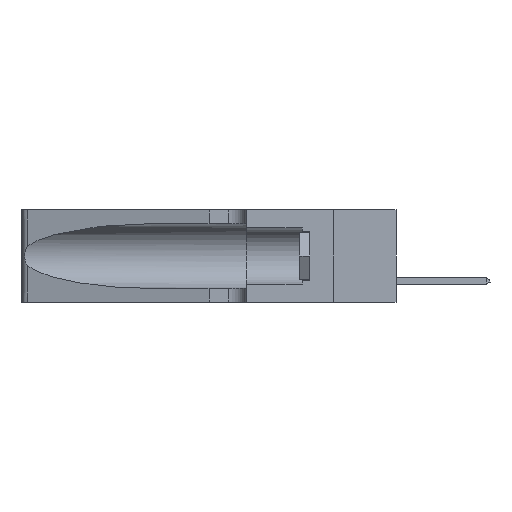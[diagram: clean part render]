
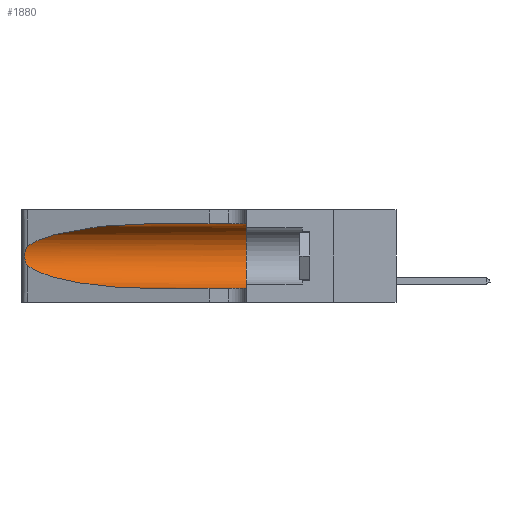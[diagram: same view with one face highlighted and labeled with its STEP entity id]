
A CAD part, left-side view. The second image highlights one B-rep face of the part: STEP entity #1880.
In plain terms, the highlighted cylindrical face has radius 3.308 mm (diameter 6.617 mm), a partial arc.
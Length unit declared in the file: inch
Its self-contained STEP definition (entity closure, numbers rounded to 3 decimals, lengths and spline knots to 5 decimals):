
#210 = CARTESIAN_POINT ( 'NONE',  ( 0.25854, 1.2359, 0.20912 ) ) ;
#938 = CARTESIAN_POINT ( 'NONE',  ( 0.2373, 1.15595, 0.08982 ) ) ;
#1553 = CARTESIAN_POINT ( 'NONE',  ( 0.1305, 1.61858, 0.31525 ) ) ;
#1868 = CARTESIAN_POINT ( 'NONE',  ( 0.2373, 1.15595, 0.28018 ) ) ;
#1880 = ADVANCED_FACE ( 'NONE', ( #12141 ), #16455, .F. ) ;
#1918 = CARTESIAN_POINT ( 'NONE',  ( 0.25639, 1.23184, 0.21858 ) ) ;
#2345 = DIRECTION ( 'NONE',  ( 0., 1., 0. ) ) ;
#3194 = CARTESIAN_POINT ( 'NONE',  ( 0.18966, 0.96281, 0.31525 ) ) ;
#3872 = CARTESIAN_POINT ( 'NONE',  ( 0.26075, 1.23896, 0.19203 ) ) ;
#3946 = CARTESIAN_POINT ( 'NONE',  ( 0.1305, 0.72297, 0.31525 ) ) ;
#4013 = CARTESIAN_POINT ( 'NONE',  ( 0.25487, 1.22718, 0.22369 ) ) ;
#4192 = VERTEX_POINT ( 'NONE', #7986 ) ;
#4742 = CARTESIAN_POINT ( 'NONE',  ( 0.1305, 0.72297, 0.05475 ) ) ;
#5266 = VERTEX_POINT ( 'NONE', #3946 ) ;
#5398 = DIRECTION ( 'NONE',  ( 0., -1., 0. ) ) ;
#5943 = CARTESIAN_POINT ( 'NONE',  ( 0.25487, 1.22718, 0.14631 ) ) ;
#6039 = AXIS2_PLACEMENT_3D ( 'NONE', #10872, #5398, #16272 ) ;
#6084 = CIRCLE ( 'NONE', #8451, 0.13025 ) ;
#6135 = LINE ( 'NONE', #1553, #21402 ) ;
#6360 = ORIENTED_EDGE ( 'NONE', *, *, #8146, .F. ) ;
#6658 = EDGE_CURVE ( 'NONE', #5266, #4192, #6135, .T. ) ;
#6794 = EDGE_LOOP ( 'NONE', ( #16082, #9988, #8717, #17207, #6360, #14737 ) ) ;
#7507 = CARTESIAN_POINT ( 'NONE',  ( 0.1305, 0.35, 0.05475 ) ) ;
#7552 = VERTEX_POINT ( 'NONE', #5943 ) ;
#7647 = CARTESIAN_POINT ( 'NONE',  ( 0.25487, 1.22718, 0.22369 ) ) ;
#7986 = CARTESIAN_POINT ( 'NONE',  ( 0.1305, 0.35, 0.31525 ) ) ;
#8146 = EDGE_CURVE ( 'NONE', #4192, #22326, #6084, .T. ) ;
#8451 = AXIS2_PLACEMENT_3D ( 'NONE', #17171, #2345, #18948 ) ;
#8602 = CARTESIAN_POINT ( 'NONE',  ( 0.1305, 0.72297, 0.05475 ) ) ;
#8717 = ORIENTED_EDGE ( 'NONE', *, *, #10031, .T. ) ;
#9177 = DIRECTION ( 'NONE',  ( 0., -1., 0. ) ) ;
#9334 = CARTESIAN_POINT ( 'NONE',  ( 0.25639, 1.23186, 0.15144 ) ) ;
#9988 = ORIENTED_EDGE ( 'NONE', *, *, #21091, .T. ) ;
#10031 = EDGE_CURVE ( 'NONE', #7552, #16902, #17265, .T. ) ;
#10510 = CARTESIAN_POINT ( 'NONE',  ( 0.1305, 0.72297, 0.31525 ) ) ;
#10872 = CARTESIAN_POINT ( 'NONE',  ( 0.1305, 1.61858, 0.185 ) ) ;
#11239 = CARTESIAN_POINT ( 'NONE',  ( 0.26018, 1.23835, 0.19895 ) ) ;
#12141 = FACE_OUTER_BOUND ( 'NONE', #6794, .T. ) ;
#13020 = CARTESIAN_POINT ( 'NONE',  ( 0.25487, 1.22718, 0.14631 ) ) ;
#13098 = CARTESIAN_POINT ( 'NONE',  ( 0.25856, 1.23593, 0.16098 ) ) ;
#13179 = CARTESIAN_POINT ( 'NONE',  ( 0.25789, 1.23486, 0.15765 ) ) ;
#13562 = VERTEX_POINT ( 'NONE', #4013 ) ;
#13925 = EDGE_CURVE ( 'NONE', #16902, #22326, #20804, .T. ) ;
#14737 = ORIENTED_EDGE ( 'NONE', *, *, #6658, .F. ) ;
#14764 = CARTESIAN_POINT ( 'NONE',  ( 0.25487, 1.22718, 0.22369 ) ) ;
#15063 = CARTESIAN_POINT ( 'NONE',  ( 0.25787, 1.23484, 0.2124 ) ) ;
#16082 = ORIENTED_EDGE ( 'NONE', *, *, #20397, .T. ) ;
#16272 = DIRECTION ( 'NONE',  ( 0., 0., -1. ) ) ;
#16455 = CYLINDRICAL_SURFACE ( 'NONE', #6039, 0.13025 ) ;
#16592 = CARTESIAN_POINT ( 'NONE',  ( 0.26075, 1.23896, 0.178 ) ) ;
#16902 = VERTEX_POINT ( 'NONE', #8602 ) ;
#17171 = CARTESIAN_POINT ( 'NONE',  ( 0.1305, 0.35, 0.185 ) ) ;
#17207 = ORIENTED_EDGE ( 'NONE', *, *, #13925, .T. ) ;
#17265 =( BOUNDED_CURVE ( )  B_SPLINE_CURVE ( 3, ( #21235, #938, #23100, #4742 ),
 .UNSPECIFIED., .F., .T. ) 
 B_SPLINE_CURVE_WITH_KNOTS ( ( 4, 4 ),
 ( 3.44316, 4.71239 ),
 .UNSPECIFIED. ) 
 CURVE ( )  GEOMETRIC_REPRESENTATION_ITEM ( )  RATIONAL_B_SPLINE_CURVE ( ( 1., 0.87, 0.87, 1. ) ) 
 REPRESENTATION_ITEM ( '' )  );
#18948 = DIRECTION ( 'NONE',  ( 0., 0., 1. ) ) ;
#19589 = CARTESIAN_POINT ( 'NONE',  ( 0.1305, 1.61858, 0.05475 ) ) ;
#20397 = EDGE_CURVE ( 'NONE', #5266, #13562, #22238, .T. ) ;
#20429 = CARTESIAN_POINT ( 'NONE',  ( 0.26017, 1.23833, 0.17102 ) ) ;
#20804 = LINE ( 'NONE', #19589, #23736 ) ;
#21091 = EDGE_CURVE ( 'NONE', #13562, #7552, #23019, .T. ) ;
#21235 = CARTESIAN_POINT ( 'NONE',  ( 0.25487, 1.22718, 0.14631 ) ) ;
#21402 = VECTOR ( 'NONE', #22154, 39.37008 ) ;
#22154 = DIRECTION ( 'NONE',  ( 0., -1., 0. ) ) ;
#22238 =( BOUNDED_CURVE ( )  B_SPLINE_CURVE ( 3, ( #10510, #3194, #1868, #14764 ),
 .UNSPECIFIED., .F., .T. ) 
 B_SPLINE_CURVE_WITH_KNOTS ( ( 4, 4 ),
 ( 1.5708, 2.84003 ),
 .UNSPECIFIED. ) 
 CURVE ( )  GEOMETRIC_REPRESENTATION_ITEM ( )  RATIONAL_B_SPLINE_CURVE ( ( 1., 0.87, 0.87, 1. ) ) 
 REPRESENTATION_ITEM ( '' )  );
#22292 = CARTESIAN_POINT ( 'NONE',  ( 0.25555, 1.22993, 0.14849 ) ) ;
#22326 = VERTEX_POINT ( 'NONE', #7507 ) ;
#22372 = CARTESIAN_POINT ( 'NONE',  ( 0.25555, 1.22994, 0.2215 ) ) ;
#23019 = B_SPLINE_CURVE_WITH_KNOTS ( 'NONE', 3,
 ( #7647, #22372, #1918, #15063, #210, #11239, #3872, #16592, #20429, #13098, #13179, #9334, #22292, #13020 ),
 .UNSPECIFIED., .F., .F.,
 ( 4, 2, 2, 2, 2, 2, 4 ),
 ( 0., 0.00027, 0.00053, 0.00107, 0.0016, 0.00187, 0.00214 ),
 .UNSPECIFIED. ) ;
#23100 = CARTESIAN_POINT ( 'NONE',  ( 0.18966, 0.96281, 0.05475 ) ) ;
#23736 = VECTOR ( 'NONE', #9177, 39.37008 ) ;
